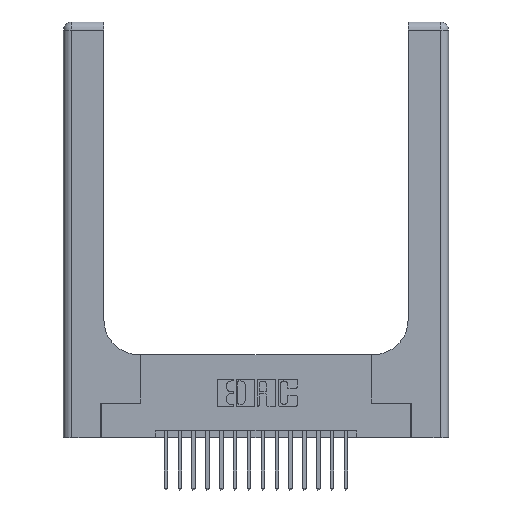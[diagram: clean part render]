
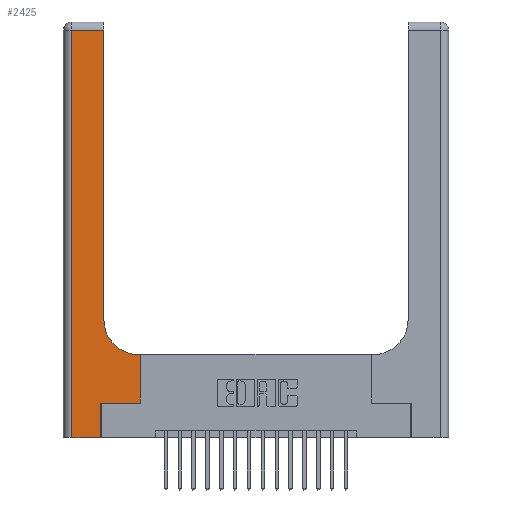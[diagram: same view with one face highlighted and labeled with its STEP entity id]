
A CAD part, top view. The second image highlights one B-rep face of the part: STEP entity #2425.
In plain terms, the highlighted planar face has unit normal (0, 0, 1).
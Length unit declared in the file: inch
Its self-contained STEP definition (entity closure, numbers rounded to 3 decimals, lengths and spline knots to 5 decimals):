
#145 = VERTEX_POINT ( 'NONE', #7407 ) ;
#565 = VERTEX_POINT ( 'NONE', #12796 ) ;
#620 = VERTEX_POINT ( 'NONE', #14674 ) ;
#765 = CARTESIAN_POINT ( 'NONE',  ( 0.06, 0., 0.37 ) ) ;
#777 = CARTESIAN_POINT ( 'NONE',  ( 0.269, 0., 0.37 ) ) ;
#1205 = DIRECTION ( 'NONE',  ( -1., 0., 0. ) ) ;
#1360 = VECTOR ( 'NONE', #13748, 39.37008 ) ;
#2242 = CARTESIAN_POINT ( 'NONE',  ( 0.2915, 3., 0.37 ) ) ;
#2380 = EDGE_CURVE ( 'NONE', #16296, #145, #5909, .T. ) ;
#2425 = ADVANCED_FACE ( 'NONE', ( #12702 ), #7352, .F. ) ;
#2896 = DIRECTION ( 'NONE',  ( 1., 0., 0. ) ) ;
#3099 = CARTESIAN_POINT ( 'NONE',  ( 0.5585, 0.25, 0.37 ) ) ;
#3102 = VECTOR ( 'NONE', #9516, 39.37008 ) ;
#3268 = ORIENTED_EDGE ( 'NONE', *, *, #17847, .T. ) ;
#3294 = EDGE_CURVE ( 'NONE', #6029, #13995, #4228, .T. ) ;
#3446 = EDGE_CURVE ( 'NONE', #13995, #8451, #19410, .T. ) ;
#3590 = LINE ( 'NONE', #17234, #3102 ) ;
#4228 = LINE ( 'NONE', #19430, #7860 ) ;
#4395 = DIRECTION ( 'NONE',  ( 0., 0., -1. ) ) ;
#4496 = DIRECTION ( 'NONE',  ( -1., 0., 0. ) ) ;
#4530 = LINE ( 'NONE', #13262, #10114 ) ;
#5909 = CIRCLE ( 'NONE', #19553, 0.25 ) ;
#5925 = CARTESIAN_POINT ( 'NONE',  ( 0.5415, 0.85, 0.37 ) ) ;
#5990 = ORIENTED_EDGE ( 'NONE', *, *, #18317, .T. ) ;
#6029 = VERTEX_POINT ( 'NONE', #765 ) ;
#6323 = ORIENTED_EDGE ( 'NONE', *, *, #11913, .T. ) ;
#6431 = LINE ( 'NONE', #3099, #7921 ) ;
#6717 = VECTOR ( 'NONE', #10692, 39.37008 ) ;
#7352 = PLANE ( 'NONE',  #13755 ) ;
#7359 = CARTESIAN_POINT ( 'NONE',  ( 0.269, 0., 0.37 ) ) ;
#7407 = CARTESIAN_POINT ( 'NONE',  ( 0.2915, 0.85, 0.37 ) ) ;
#7420 = CARTESIAN_POINT ( 'NONE',  ( 0., 3., 0.37 ) ) ;
#7465 = EDGE_CURVE ( 'NONE', #145, #565, #16579, .T. ) ;
#7647 = VERTEX_POINT ( 'NONE', #13790 ) ;
#7860 = VECTOR ( 'NONE', #10839, 39.37008 ) ;
#7921 = VECTOR ( 'NONE', #12467, 39.37008 ) ;
#7926 = ORIENTED_EDGE ( 'NONE', *, *, #8938, .T. ) ;
#8029 = CARTESIAN_POINT ( 'NONE',  ( 0.269, 0.25, 0.37 ) ) ;
#8451 = VERTEX_POINT ( 'NONE', #18661 ) ;
#8521 = EDGE_CURVE ( 'NONE', #565, #7647, #3590, .T. ) ;
#8938 = EDGE_CURVE ( 'NONE', #10737, #16296, #4530, .T. ) ;
#9516 = DIRECTION ( 'NONE',  ( -1., 0., 0. ) ) ;
#9846 = ORIENTED_EDGE ( 'NONE', *, *, #7465, .T. ) ;
#10114 = VECTOR ( 'NONE', #4496, 39.37008 ) ;
#10548 = DIRECTION ( 'NONE',  ( 0., 1., 0. ) ) ;
#10692 = DIRECTION ( 'NONE',  ( 0., -1., 0. ) ) ;
#10737 = VERTEX_POINT ( 'NONE', #15962 ) ;
#10839 = DIRECTION ( 'NONE',  ( 1., 0., 0. ) ) ;
#10847 = LINE ( 'NONE', #16731, #6717 ) ;
#11913 = EDGE_CURVE ( 'NONE', #8451, #620, #13676, .T. ) ;
#12012 = VECTOR ( 'NONE', #16162, 39.37008 ) ;
#12235 = ORIENTED_EDGE ( 'NONE', *, *, #3446, .T. ) ;
#12467 = DIRECTION ( 'NONE',  ( 0., 1., 0. ) ) ;
#12532 = ORIENTED_EDGE ( 'NONE', *, *, #8521, .T. ) ;
#12702 = FACE_OUTER_BOUND ( 'NONE', #14667, .T. ) ;
#12796 = CARTESIAN_POINT ( 'NONE',  ( 0.2915, 2.94, 0.37 ) ) ;
#13262 = CARTESIAN_POINT ( 'NONE',  ( 0.2915, 0.6, 0.37 ) ) ;
#13676 = LINE ( 'NONE', #8029, #1360 ) ;
#13748 = DIRECTION ( 'NONE',  ( 1., 0., 0. ) ) ;
#13755 = AXIS2_PLACEMENT_3D ( 'NONE', #7420, #15105, #1205 ) ;
#13790 = CARTESIAN_POINT ( 'NONE',  ( 0.06, 2.94, 0.37 ) ) ;
#13995 = VERTEX_POINT ( 'NONE', #777 ) ;
#14667 = EDGE_LOOP ( 'NONE', ( #9846, #12532, #3268, #15047, #12235, #6323, #5990, #7926, #16684 ) ) ;
#14674 = CARTESIAN_POINT ( 'NONE',  ( 0.5585, 0.25, 0.37 ) ) ;
#15047 = ORIENTED_EDGE ( 'NONE', *, *, #3294, .T. ) ;
#15105 = DIRECTION ( 'NONE',  ( 0., 0., -1. ) ) ;
#15888 = CARTESIAN_POINT ( 'NONE',  ( 0.5415, 0.6, 0.37 ) ) ;
#15962 = CARTESIAN_POINT ( 'NONE',  ( 0.5585, 0.6, 0.37 ) ) ;
#16046 = VECTOR ( 'NONE', #10548, 39.37008 ) ;
#16162 = DIRECTION ( 'NONE',  ( 0., 1., 0. ) ) ;
#16296 = VERTEX_POINT ( 'NONE', #15888 ) ;
#16579 = LINE ( 'NONE', #2242, #12012 ) ;
#16684 = ORIENTED_EDGE ( 'NONE', *, *, #2380, .T. ) ;
#16731 = CARTESIAN_POINT ( 'NONE',  ( 0.06, 3., 0.37 ) ) ;
#17234 = CARTESIAN_POINT ( 'NONE',  ( 0., 2.94, 0.37 ) ) ;
#17847 = EDGE_CURVE ( 'NONE', #7647, #6029, #10847, .T. ) ;
#18317 = EDGE_CURVE ( 'NONE', #620, #10737, #6431, .T. ) ;
#18661 = CARTESIAN_POINT ( 'NONE',  ( 0.269, 0.25, 0.37 ) ) ;
#19410 = LINE ( 'NONE', #7359, #16046 ) ;
#19430 = CARTESIAN_POINT ( 'NONE',  ( 0., 0., 0.37 ) ) ;
#19553 = AXIS2_PLACEMENT_3D ( 'NONE', #5925, #4395, #2896 ) ;
